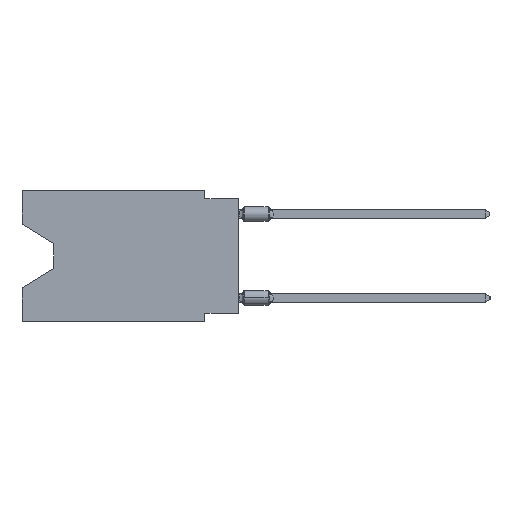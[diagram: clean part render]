
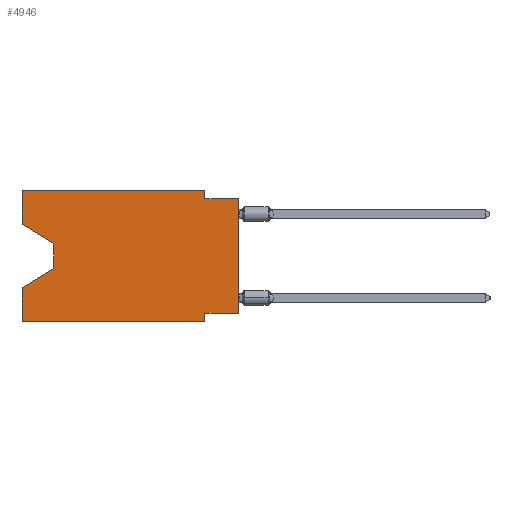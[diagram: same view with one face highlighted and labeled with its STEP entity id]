
A CAD part, left-side view. The second image highlights one B-rep face of the part: STEP entity #4946.
In plain terms, the highlighted planar face has unit normal (-1, 0, 0).
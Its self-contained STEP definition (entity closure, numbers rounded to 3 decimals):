
#887 = VECTOR ( 'NONE', #10356, 1000. ) ;
#1713 = EDGE_CURVE ( 'NONE', #32210, #25642, #38641, .T. ) ;
#2801 = ORIENTED_EDGE ( 'NONE', *, *, #25500, .T. ) ;
#2807 = VECTOR ( 'NONE', #3244, 1000. ) ;
#3244 = DIRECTION ( 'NONE',  ( 0., 0., -1. ) ) ;
#4946 = ADVANCED_FACE ( 'NONE', ( #38873 ), #10451, .F. ) ;
#5470 = EDGE_CURVE ( 'NONE', #37258, #18474, #25041, .T. ) ;
#5756 = EDGE_LOOP ( 'NONE', ( #13482, #2801, #23068, #33754, #5956, #31906, #8872, #37632, #14008, #21282, #19034, #38295 ) ) ;
#5956 = ORIENTED_EDGE ( 'NONE', *, *, #5470, .T. ) ;
#6413 = DIRECTION ( 'NONE',  ( 0., -1., 0. ) ) ;
#6538 = CARTESIAN_POINT ( 'NONE',  ( 0., 2.54, -9.906 ) ) ;
#6769 = CARTESIAN_POINT ( 'NONE',  ( 0., 16.383, -2.546 ) ) ;
#7100 = CARTESIAN_POINT ( 'NONE',  ( 0., 0., 0. ) ) ;
#7335 = DIRECTION ( 'NONE',  ( 1., 0., 0. ) ) ;
#8140 = EDGE_CURVE ( 'NONE', #13784, #25642, #25316, .T. ) ;
#8349 = EDGE_CURVE ( 'NONE', #37026, #18433, #25555, .T. ) ;
#8872 = ORIENTED_EDGE ( 'NONE', *, *, #12341, .F. ) ;
#9984 = DIRECTION ( 'NONE',  ( 0., -1., 0. ) ) ;
#10356 = DIRECTION ( 'NONE',  ( 0., 0., 1. ) ) ;
#10451 = PLANE ( 'NONE',  #32184 ) ;
#11512 = VECTOR ( 'NONE', #36988, 1000. ) ;
#11579 = DIRECTION ( 'NONE',  ( 0., -1., 0. ) ) ;
#11753 = VECTOR ( 'NONE', #23034, 1000. ) ;
#12049 = LINE ( 'NONE', #31334, #25160 ) ;
#12125 = CARTESIAN_POINT ( 'NONE',  ( 0., 13.97, -5.893 ) ) ;
#12254 = DIRECTION ( 'NONE',  ( 0., 0., 1. ) ) ;
#12341 = EDGE_CURVE ( 'NONE', #32210, #29099, #26508, .T. ) ;
#12693 = CARTESIAN_POINT ( 'NONE',  ( 0., 0., -9.271 ) ) ;
#13482 = ORIENTED_EDGE ( 'NONE', *, *, #21638, .T. ) ;
#13784 = VERTEX_POINT ( 'NONE', #31107 ) ;
#14008 = ORIENTED_EDGE ( 'NONE', *, *, #8140, .F. ) ;
#14573 = EDGE_CURVE ( 'NONE', #29099, #18474, #39681, .T. ) ;
#16311 = CARTESIAN_POINT ( 'NONE',  ( 0., 13.97, -4.013 ) ) ;
#16805 = CARTESIAN_POINT ( 'NONE',  ( 0., 2.54, 0. ) ) ;
#17083 = DIRECTION ( 'NONE',  ( 0., 0., -1. ) ) ;
#17961 = CARTESIAN_POINT ( 'NONE',  ( 0., 2.54, -9.271 ) ) ;
#18433 = VERTEX_POINT ( 'NONE', #34361 ) ;
#18474 = VERTEX_POINT ( 'NONE', #6538 ) ;
#18674 = DIRECTION ( 'NONE',  ( 0., -0.855, -0.519 ) ) ;
#19033 = VECTOR ( 'NONE', #6413, 1000. ) ;
#19034 = ORIENTED_EDGE ( 'NONE', *, *, #8349, .F. ) ;
#19263 = CARTESIAN_POINT ( 'NONE',  ( 0., 16.383, 0. ) ) ;
#19651 = CARTESIAN_POINT ( 'NONE',  ( 0., 0., -9.271 ) ) ;
#20071 = CARTESIAN_POINT ( 'NONE',  ( 0., 16.383, -9.906 ) ) ;
#20113 = LINE ( 'NONE', #16805, #11753 ) ;
#21282 = ORIENTED_EDGE ( 'NONE', *, *, #39659, .F. ) ;
#21340 = CARTESIAN_POINT ( 'NONE',  ( 0., 16.383, 0. ) ) ;
#21489 = EDGE_CURVE ( 'NONE', #34388, #37026, #12049, .T. ) ;
#21638 = EDGE_CURVE ( 'NONE', #34388, #39003, #28012, .T. ) ;
#22939 = LINE ( 'NONE', #16311, #2807 ) ;
#23034 = DIRECTION ( 'NONE',  ( 0., 0., -1. ) ) ;
#23068 = ORIENTED_EDGE ( 'NONE', *, *, #25575, .T. ) ;
#23096 = CARTESIAN_POINT ( 'NONE',  ( 0., 16.383, 0. ) ) ;
#23555 = CARTESIAN_POINT ( 'NONE',  ( 0., 13.97, -5.893 ) ) ;
#24188 = VERTEX_POINT ( 'NONE', #12125 ) ;
#24226 = CARTESIAN_POINT ( 'NONE',  ( 0., 16.383, -7.36 ) ) ;
#25041 = LINE ( 'NONE', #39994, #26920 ) ;
#25160 = VECTOR ( 'NONE', #12254, 1000. ) ;
#25316 = LINE ( 'NONE', #37973, #19033 ) ;
#25500 = EDGE_CURVE ( 'NONE', #39003, #24188, #22939, .T. ) ;
#25555 = LINE ( 'NONE', #35293, #29665 ) ;
#25575 = EDGE_CURVE ( 'NONE', #24188, #26298, #29599, .T. ) ;
#25642 = VERTEX_POINT ( 'NONE', #33313 ) ;
#26210 = EDGE_CURVE ( 'NONE', #37258, #26298, #28621, .T. ) ;
#26298 = VERTEX_POINT ( 'NONE', #24226 ) ;
#26508 = LINE ( 'NONE', #19651, #26548 ) ;
#26548 = VECTOR ( 'NONE', #38962, 1000. ) ;
#26605 = DIRECTION ( 'NONE',  ( 0., 0., 1. ) ) ;
#26920 = VECTOR ( 'NONE', #11579, 1000. ) ;
#27650 = CARTESIAN_POINT ( 'NONE',  ( 0., 2.54, -9.906 ) ) ;
#28012 = LINE ( 'NONE', #34652, #31116 ) ;
#28621 = LINE ( 'NONE', #19263, #887 ) ;
#29099 = VERTEX_POINT ( 'NONE', #17961 ) ;
#29599 = LINE ( 'NONE', #23555, #37988 ) ;
#29665 = VECTOR ( 'NONE', #9984, 1000. ) ;
#30001 = CARTESIAN_POINT ( 'NONE',  ( 0., 13.97, -4.013 ) ) ;
#30213 = DIRECTION ( 'NONE',  ( 0., 0.855, -0.519 ) ) ;
#31107 = CARTESIAN_POINT ( 'NONE',  ( 0., 2.54, -0.635 ) ) ;
#31116 = VECTOR ( 'NONE', #18674, 1000. ) ;
#31334 = CARTESIAN_POINT ( 'NONE',  ( 0., 16.383, 0. ) ) ;
#31340 = VECTOR ( 'NONE', #26605, 1000. ) ;
#31906 = ORIENTED_EDGE ( 'NONE', *, *, #14573, .F. ) ;
#32184 = AXIS2_PLACEMENT_3D ( 'NONE', #23096, #7335, #17083 ) ;
#32210 = VERTEX_POINT ( 'NONE', #12693 ) ;
#33313 = CARTESIAN_POINT ( 'NONE',  ( 0., 0., -0.635 ) ) ;
#33754 = ORIENTED_EDGE ( 'NONE', *, *, #26210, .F. ) ;
#34361 = CARTESIAN_POINT ( 'NONE',  ( 0., 2.54, 0. ) ) ;
#34388 = VERTEX_POINT ( 'NONE', #6769 ) ;
#34652 = CARTESIAN_POINT ( 'NONE',  ( 0., 16.383, -2.546 ) ) ;
#35293 = CARTESIAN_POINT ( 'NONE',  ( 0., 16.383, 0. ) ) ;
#36988 = DIRECTION ( 'NONE',  ( 0., 0., -1. ) ) ;
#37026 = VERTEX_POINT ( 'NONE', #21340 ) ;
#37258 = VERTEX_POINT ( 'NONE', #20071 ) ;
#37632 = ORIENTED_EDGE ( 'NONE', *, *, #1713, .T. ) ;
#37973 = CARTESIAN_POINT ( 'NONE',  ( 0., 0., -0.635 ) ) ;
#37988 = VECTOR ( 'NONE', #30213, 1000. ) ;
#38295 = ORIENTED_EDGE ( 'NONE', *, *, #21489, .F. ) ;
#38641 = LINE ( 'NONE', #7100, #31340 ) ;
#38873 = FACE_OUTER_BOUND ( 'NONE', #5756, .T. ) ;
#38962 = DIRECTION ( 'NONE',  ( 0., 1., 0. ) ) ;
#39003 = VERTEX_POINT ( 'NONE', #30001 ) ;
#39659 = EDGE_CURVE ( 'NONE', #18433, #13784, #20113, .T. ) ;
#39681 = LINE ( 'NONE', #27650, #11512 ) ;
#39994 = CARTESIAN_POINT ( 'NONE',  ( 0., 16.383, -9.906 ) ) ;
